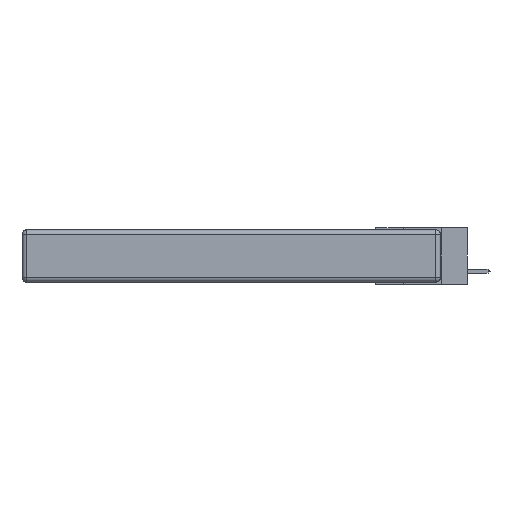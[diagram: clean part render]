
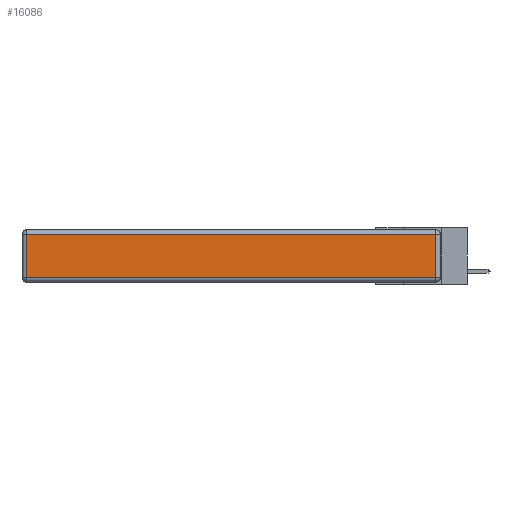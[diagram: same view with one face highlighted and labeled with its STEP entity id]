
A CAD part, left-side view. The second image highlights one B-rep face of the part: STEP entity #16086.
In plain terms, the highlighted planar face has unit normal (-1, 0, 0).
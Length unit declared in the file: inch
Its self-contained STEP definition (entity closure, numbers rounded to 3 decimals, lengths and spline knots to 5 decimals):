
#1533 = CARTESIAN_POINT ( 'NONE',  ( 0., 2.72, -0.343 ) ) ;
#1800 = EDGE_CURVE ( 'NONE', #15631, #6294, #15638, .T. ) ;
#1825 = CARTESIAN_POINT ( 'NONE',  ( 0., 0., -0.343 ) ) ;
#1998 = ORIENTED_EDGE ( 'NONE', *, *, #6977, .T. ) ;
#2072 = CARTESIAN_POINT ( 'NONE',  ( 0., 0.03, -0.313 ) ) ;
#2488 = LINE ( 'NONE', #13882, #17610 ) ;
#2627 = DIRECTION ( 'NONE',  ( 0., 1., 0. ) ) ;
#3508 = AXIS2_PLACEMENT_3D ( 'NONE', #1825, #7475, #9442 ) ;
#3612 = DIRECTION ( 'NONE',  ( 0., -1., 0. ) ) ;
#3628 = PLANE ( 'NONE',  #3508 ) ;
#3892 = ORIENTED_EDGE ( 'NONE', *, *, #24111, .T. ) ;
#5233 = VECTOR ( 'NONE', #19308, 39.37008 ) ;
#5752 = ORIENTED_EDGE ( 'NONE', *, *, #1800, .T. ) ;
#6294 = VERTEX_POINT ( 'NONE', #22714 ) ;
#6977 = EDGE_CURVE ( 'NONE', #6294, #24426, #8900, .T. ) ;
#7475 = DIRECTION ( 'NONE',  ( -1., 0., 0. ) ) ;
#8900 = LINE ( 'NONE', #16422, #14775 ) ;
#8973 = CARTESIAN_POINT ( 'NONE',  ( 0., 0.03, -0.343 ) ) ;
#9305 = VERTEX_POINT ( 'NONE', #14527 ) ;
#9442 = DIRECTION ( 'NONE',  ( 0., 0., 1. ) ) ;
#9852 = LINE ( 'NONE', #1533, #5233 ) ;
#13151 = CARTESIAN_POINT ( 'NONE',  ( 0., 2.72, -0.03 ) ) ;
#13882 = CARTESIAN_POINT ( 'NONE',  ( 0., 0., -0.313 ) ) ;
#14045 = EDGE_LOOP ( 'NONE', ( #21460, #5752, #1998, #3892 ) ) ;
#14527 = CARTESIAN_POINT ( 'NONE',  ( 0., 2.72, -0.313 ) ) ;
#14775 = VECTOR ( 'NONE', #2627, 39.37008 ) ;
#15185 = DIRECTION ( 'NONE',  ( 0., 0., 1. ) ) ;
#15631 = VERTEX_POINT ( 'NONE', #2072 ) ;
#15638 = LINE ( 'NONE', #8973, #22433 ) ;
#15728 = FACE_OUTER_BOUND ( 'NONE', #14045, .T. ) ;
#16086 = ADVANCED_FACE ( 'NONE', ( #15728 ), #3628, .T. ) ;
#16422 = CARTESIAN_POINT ( 'NONE',  ( 0., 2.75, -0.03 ) ) ;
#16707 = EDGE_CURVE ( 'NONE', #9305, #15631, #2488, .T. ) ;
#17610 = VECTOR ( 'NONE', #3612, 39.37008 ) ;
#19308 = DIRECTION ( 'NONE',  ( 0., 0., -1. ) ) ;
#21460 = ORIENTED_EDGE ( 'NONE', *, *, #16707, .T. ) ;
#22433 = VECTOR ( 'NONE', #15185, 39.37008 ) ;
#22714 = CARTESIAN_POINT ( 'NONE',  ( 0., 0.03, -0.03 ) ) ;
#24111 = EDGE_CURVE ( 'NONE', #24426, #9305, #9852, .T. ) ;
#24426 = VERTEX_POINT ( 'NONE', #13151 ) ;
